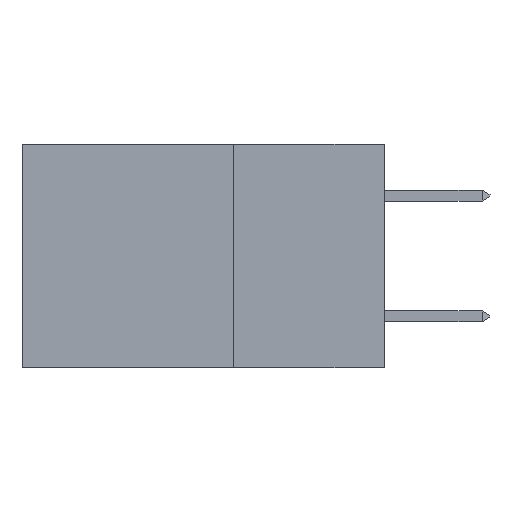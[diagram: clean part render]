
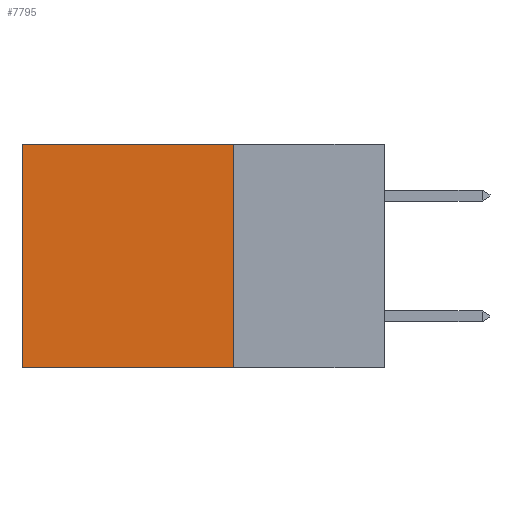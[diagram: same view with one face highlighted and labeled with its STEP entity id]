
A CAD part, left-side view. The second image highlights one B-rep face of the part: STEP entity #7795.
In plain terms, the highlighted planar face has unit normal (-1, 0, 0).
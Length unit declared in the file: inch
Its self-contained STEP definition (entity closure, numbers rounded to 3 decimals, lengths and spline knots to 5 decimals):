
#29 = VERTEX_POINT ( 'NONE', #684 ) ;
#70 = VECTOR ( 'NONE', #6076, 39.37008 ) ;
#684 = CARTESIAN_POINT ( 'NONE',  ( 0.2875, 0.6, 0. ) ) ;
#818 = LINE ( 'NONE', #5957, #6232 ) ;
#928 = CARTESIAN_POINT ( 'NONE',  ( 0.2875, 0.25, 0. ) ) ;
#941 = ORIENTED_EDGE ( 'NONE', *, *, #957, .F. ) ;
#957 = EDGE_CURVE ( 'NONE', #4873, #1691, #2205, .T. ) ;
#1100 = CARTESIAN_POINT ( 'NONE',  ( 0.2875, 0.25, 0. ) ) ;
#1236 = CARTESIAN_POINT ( 'NONE',  ( 0.2875, 0.25, 0. ) ) ;
#1366 = VECTOR ( 'NONE', #6414, 39.37008 ) ;
#1379 = EDGE_CURVE ( 'NONE', #29, #1691, #818, .T. ) ;
#1691 = VERTEX_POINT ( 'NONE', #9079 ) ;
#1957 = VERTEX_POINT ( 'NONE', #1100 ) ;
#2170 = ORIENTED_EDGE ( 'NONE', *, *, #9428, .T. ) ;
#2205 = LINE ( 'NONE', #9340, #70 ) ;
#2910 = DIRECTION ( 'NONE',  ( 0., 1., 0. ) ) ;
#4643 = AXIS2_PLACEMENT_3D ( 'NONE', #9168, #7562, #6762 ) ;
#4873 = VERTEX_POINT ( 'NONE', #10174 ) ;
#5213 = DIRECTION ( 'NONE',  ( 0., 0., -1. ) ) ;
#5957 = CARTESIAN_POINT ( 'NONE',  ( 0.2875, 0.6, 0. ) ) ;
#5985 = PLANE ( 'NONE',  #4643 ) ;
#6076 = DIRECTION ( 'NONE',  ( 0., 1., 0. ) ) ;
#6232 = VECTOR ( 'NONE', #5213, 39.37008 ) ;
#6414 = DIRECTION ( 'NONE',  ( 0., 0., -1. ) ) ;
#6692 = ORIENTED_EDGE ( 'NONE', *, *, #7456, .F. ) ;
#6721 = ORIENTED_EDGE ( 'NONE', *, *, #1379, .T. ) ;
#6762 = DIRECTION ( 'NONE',  ( 0., 0., -1. ) ) ;
#7456 = EDGE_CURVE ( 'NONE', #1957, #4873, #7666, .T. ) ;
#7562 = DIRECTION ( 'NONE',  ( 1., 0., 0. ) ) ;
#7666 = LINE ( 'NONE', #928, #1366 ) ;
#7755 = LINE ( 'NONE', #1236, #7986 ) ;
#7795 = ADVANCED_FACE ( 'NONE', ( #9177 ), #5985, .F. ) ;
#7986 = VECTOR ( 'NONE', #2910, 39.37008 ) ;
#8965 = EDGE_LOOP ( 'NONE', ( #6721, #941, #6692, #2170 ) ) ;
#9079 = CARTESIAN_POINT ( 'NONE',  ( 0.2875, 0.6, -0.37 ) ) ;
#9168 = CARTESIAN_POINT ( 'NONE',  ( 0.2875, 0.25, 0. ) ) ;
#9177 = FACE_OUTER_BOUND ( 'NONE', #8965, .T. ) ;
#9340 = CARTESIAN_POINT ( 'NONE',  ( 0.2875, 0.25, -0.37 ) ) ;
#9428 = EDGE_CURVE ( 'NONE', #1957, #29, #7755, .T. ) ;
#10174 = CARTESIAN_POINT ( 'NONE',  ( 0.2875, 0.25, -0.37 ) ) ;
